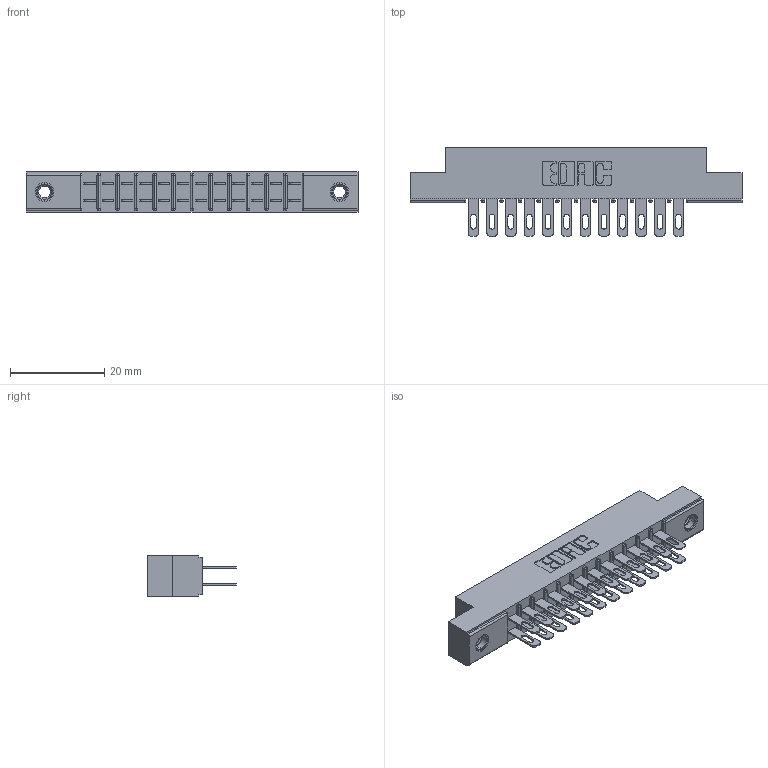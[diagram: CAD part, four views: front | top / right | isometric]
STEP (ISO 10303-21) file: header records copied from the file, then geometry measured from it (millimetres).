
FILE_DESCRIPTION (( 'STEP AP203' ), '1' );
FILE_NAME ('355-024-500-507.STEP', '2019-09-11T04:35:34', ( '' ), ( '' ), 'SwSTEP 2.0', 'SolidWorks 2016', '' );
FILE_SCHEMA (( 'CONFIG_CONTROL_DESIGN' ));
Length unit declared in the file: inch
Products named in the file (4): 355-024-500-507; 305-290-001_500; 345-250-001_345-250-005-103; 305 Part_.156 Dia
Assembly tree (27 placements, depth 2):
  355-024-500-507
    305 Part_.156 Dia
    305-290-001_500  x24
    345-250-001_345-250-005-103  x2
Bounding box: 70.56 x 18.85 x 8.71 mm (x, y, z)
Volume: 4328.4 mm3; surface area: 8438.9 mm2
Topology: 27 solids, 27 shells, 1376 faces, 3896 edges, 2524 vertices
Faces by surface type: plane 772, cylinder 540, sphere 48, cone 12, torus 4
Entity records: 17852 total; most frequent: CARTESIAN_POINT 2937, ORIENTED_EDGE 2904, DIRECTION 2878, EDGE_CURVE 1452, LINE 1136, VECTOR 1136, VERTEX_POINT 930, AXIS2_PLACEMENT_3D 871
